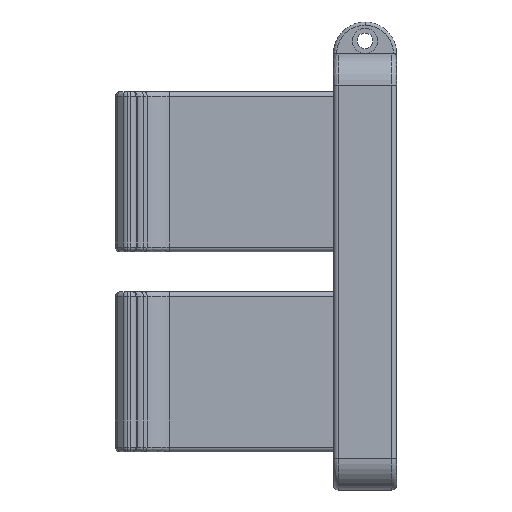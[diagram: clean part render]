
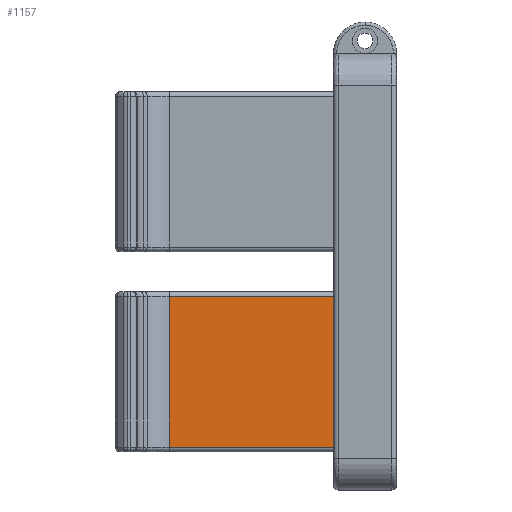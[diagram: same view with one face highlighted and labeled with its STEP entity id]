
A CAD part, left-side view. The second image highlights one B-rep face of the part: STEP entity #1157.
In plain terms, the highlighted planar face has unit normal (-1, 0, 0).
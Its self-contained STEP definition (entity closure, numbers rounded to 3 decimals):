
#394 = AXIS2_PLACEMENT_3D ( 'NONE', #2816, #6531, #3346 ) ;
#430 = CARTESIAN_POINT ( 'NONE',  ( 34.098, 0., -3.925 ) ) ;
#437 = CARTESIAN_POINT ( 'NONE',  ( 34.098, 7.884, -3.925 ) ) ;
#466 = FACE_OUTER_BOUND ( 'NONE', #6269, .T. ) ;
#577 = CARTESIAN_POINT ( 'NONE',  ( 34.098, 0., -27.825 ) ) ;
#702 = ORIENTED_EDGE ( 'NONE', *, *, #1095, .T. ) ;
#951 = DIRECTION ( 'NONE',  ( 0., 1., 0. ) ) ;
#1093 = ORIENTED_EDGE ( 'NONE', *, *, #6720, .T. ) ;
#1095 = EDGE_CURVE ( 'NONE', #3667, #6485, #6285, .T. ) ;
#1106 = DIRECTION ( 'NONE',  ( 0., -1., 0. ) ) ;
#1157 = ADVANCED_FACE ( 'NONE', ( #466 ), #1785, .F. ) ;
#1340 = LINE ( 'NONE', #1371, #4137 ) ;
#1371 = CARTESIAN_POINT ( 'NONE',  ( 34.098, 7.884, -34.631 ) ) ;
#1785 = PLANE ( 'NONE',  #394 ) ;
#1953 = VECTOR ( 'NONE', #2517, 1000. ) ;
#2371 = LINE ( 'NONE', #430, #3265 ) ;
#2517 = DIRECTION ( 'NONE',  ( 0., 0., -1. ) ) ;
#2816 = CARTESIAN_POINT ( 'NONE',  ( 34.098, 0., -34.631 ) ) ;
#3265 = VECTOR ( 'NONE', #951, 1000. ) ;
#3346 = DIRECTION ( 'NONE',  ( 0., 0., 1. ) ) ;
#3667 = VERTEX_POINT ( 'NONE', #6261 ) ;
#3951 = ORIENTED_EDGE ( 'NONE', *, *, #4656, .F. ) ;
#4137 = VECTOR ( 'NONE', #5039, 1000. ) ;
#4656 = EDGE_CURVE ( 'NONE', #6698, #6485, #1340, .T. ) ;
#4711 = VERTEX_POINT ( 'NONE', #5652 ) ;
#4855 = VECTOR ( 'NONE', #1106, 1000. ) ;
#5021 = CARTESIAN_POINT ( 'NONE',  ( 34.098, 7.884, -27.825 ) ) ;
#5039 = DIRECTION ( 'NONE',  ( 0., 0., -1. ) ) ;
#5172 = CARTESIAN_POINT ( 'NONE',  ( 34.098, 41.413, -34.631 ) ) ;
#5263 = ORIENTED_EDGE ( 'NONE', *, *, #5415, .T. ) ;
#5415 = EDGE_CURVE ( 'NONE', #6698, #4711, #2371, .T. ) ;
#5652 = CARTESIAN_POINT ( 'NONE',  ( 34.098, 41.413, -3.925 ) ) ;
#5981 = LINE ( 'NONE', #5172, #1953 ) ;
#6261 = CARTESIAN_POINT ( 'NONE',  ( 34.098, 41.413, -27.825 ) ) ;
#6269 = EDGE_LOOP ( 'NONE', ( #5263, #1093, #702, #3951 ) ) ;
#6285 = LINE ( 'NONE', #577, #4855 ) ;
#6485 = VERTEX_POINT ( 'NONE', #5021 ) ;
#6531 = DIRECTION ( 'NONE',  ( 1., 0., 0. ) ) ;
#6698 = VERTEX_POINT ( 'NONE', #437 ) ;
#6720 = EDGE_CURVE ( 'NONE', #4711, #3667, #5981, .T. ) ;
